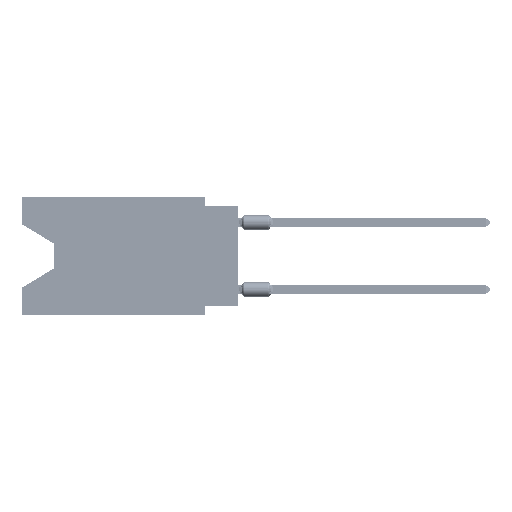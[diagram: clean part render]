
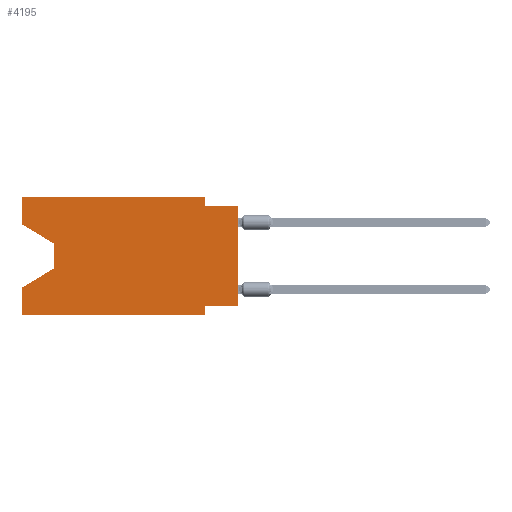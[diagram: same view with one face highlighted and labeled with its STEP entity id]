
A CAD part, left-side view. The second image highlights one B-rep face of the part: STEP entity #4195.
In plain terms, the highlighted planar face has unit normal (-1, 0, 0).
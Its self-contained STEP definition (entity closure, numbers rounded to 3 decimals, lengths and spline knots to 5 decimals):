
#180 = DIRECTION ( 'NONE',  ( 0., -1., 0. ) ) ;
#214 = CARTESIAN_POINT ( 'NONE',  ( 0., 0.645, 0. ) ) ;
#502 = VERTEX_POINT ( 'NONE', #81972 ) ;
#677 = CARTESIAN_POINT ( 'NONE',  ( 0., 0.645, 0. ) ) ;
#2308 = CARTESIAN_POINT ( 'NONE',  ( 0., 0.1, -0.35 ) ) ;
#4195 = ADVANCED_FACE ( 'NONE', ( #60947 ), #52867, .F. ) ;
#5305 = CARTESIAN_POINT ( 'NONE',  ( 0., 0.645, 0. ) ) ;
#5791 = CARTESIAN_POINT ( 'NONE',  ( 0., 0.1, 0. ) ) ;
#6716 = ORIENTED_EDGE ( 'NONE', *, *, #38894, .F. ) ;
#7738 = EDGE_CURVE ( 'NONE', #95306, #88112, #59774, .T. ) ;
#8218 = VECTOR ( 'NONE', #21999, 39.37008 ) ;
#10416 = DIRECTION ( 'NONE',  ( 0., 0., -1. ) ) ;
#10576 = DIRECTION ( 'NONE',  ( 0., -1., 0. ) ) ;
#14417 = LINE ( 'NONE', #21009, #8218 ) ;
#14703 = EDGE_CURVE ( 'NONE', #55074, #41310, #25759, .T. ) ;
#16935 = ORIENTED_EDGE ( 'NONE', *, *, #26205, .T. ) ;
#18198 = LINE ( 'NONE', #49082, #52722 ) ;
#19503 = CARTESIAN_POINT ( 'NONE',  ( 0., 0.55, -0.212 ) ) ;
#21009 = CARTESIAN_POINT ( 'NONE',  ( 0., 0., -0.025 ) ) ;
#21348 = VECTOR ( 'NONE', #34677, 39.37008 ) ;
#21877 = VECTOR ( 'NONE', #88102, 39.37008 ) ;
#21999 = DIRECTION ( 'NONE',  ( 0., -1., 0. ) ) ;
#23014 = CARTESIAN_POINT ( 'NONE',  ( 0., 0.645, -0.35 ) ) ;
#25307 = LINE ( 'NONE', #57171, #21877 ) ;
#25759 = LINE ( 'NONE', #79935, #85732 ) ;
#26205 = EDGE_CURVE ( 'NONE', #72368, #79145, #18198, .T. ) ;
#26707 = VECTOR ( 'NONE', #10416, 39.37008 ) ;
#26899 = CARTESIAN_POINT ( 'NONE',  ( 0., 0.1, 0. ) ) ;
#32857 = DIRECTION ( 'NONE',  ( 0., 0., 1. ) ) ;
#33071 = EDGE_CURVE ( 'NONE', #60863, #79145, #14417, .T. ) ;
#34677 = DIRECTION ( 'NONE',  ( 0., 0., -1. ) ) ;
#36198 = VERTEX_POINT ( 'NONE', #26899 ) ;
#36480 = CARTESIAN_POINT ( 'NONE',  ( 0., 0.645, -0.08025 ) ) ;
#37240 = CARTESIAN_POINT ( 'NONE',  ( 0., 0.645, -0.08025 ) ) ;
#37495 = DIRECTION ( 'NONE',  ( 0., -0.855, -0.519 ) ) ;
#37634 = VERTEX_POINT ( 'NONE', #64694 ) ;
#38363 = EDGE_CURVE ( 'NONE', #72368, #89957, #78567, .T. ) ;
#38894 = EDGE_CURVE ( 'NONE', #95306, #37634, #80423, .T. ) ;
#40051 = CARTESIAN_POINT ( 'NONE',  ( 0., 0., -0.325 ) ) ;
#41310 = VERTEX_POINT ( 'NONE', #59837 ) ;
#42285 = DIRECTION ( 'NONE',  ( 0., 0., 1. ) ) ;
#49082 = CARTESIAN_POINT ( 'NONE',  ( 0., 0., 0. ) ) ;
#49343 = EDGE_CURVE ( 'NONE', #55074, #502, #65061, .T. ) ;
#49981 = CARTESIAN_POINT ( 'NONE',  ( 0., 0.55, -0.138 ) ) ;
#52722 = VECTOR ( 'NONE', #74370, 39.37008 ) ;
#52867 = PLANE ( 'NONE',  #79318 ) ;
#53057 = CARTESIAN_POINT ( 'NONE',  ( 0., 0.1, -0.025 ) ) ;
#53303 = VECTOR ( 'NONE', #42285, 39.37008 ) ;
#53385 = ORIENTED_EDGE ( 'NONE', *, *, #49343, .F. ) ;
#54950 = ORIENTED_EDGE ( 'NONE', *, *, #76757, .T. ) ;
#55024 = ORIENTED_EDGE ( 'NONE', *, *, #33071, .F. ) ;
#55074 = VERTEX_POINT ( 'NONE', #23014 ) ;
#55363 = CARTESIAN_POINT ( 'NONE',  ( 0., 0.55, -0.212 ) ) ;
#55741 = DIRECTION ( 'NONE',  ( 0., 0., -1. ) ) ;
#56237 = ORIENTED_EDGE ( 'NONE', *, *, #38363, .F. ) ;
#56540 = VECTOR ( 'NONE', #180, 39.37008 ) ;
#56626 = CARTESIAN_POINT ( 'NONE',  ( 0., 0.645, 0. ) ) ;
#57171 = CARTESIAN_POINT ( 'NONE',  ( 0., 0.55, -0.138 ) ) ;
#58378 = VERTEX_POINT ( 'NONE', #55363 ) ;
#59080 = CARTESIAN_POINT ( 'NONE',  ( 0., 0., -0.325 ) ) ;
#59774 = LINE ( 'NONE', #36480, #72070 ) ;
#59837 = CARTESIAN_POINT ( 'NONE',  ( 0., 0.1, -0.35 ) ) ;
#60863 = VERTEX_POINT ( 'NONE', #53057 ) ;
#60910 = LINE ( 'NONE', #677, #56540 ) ;
#60947 = FACE_OUTER_BOUND ( 'NONE', #99582, .T. ) ;
#62619 = ORIENTED_EDGE ( 'NONE', *, *, #73472, .F. ) ;
#63772 = ORIENTED_EDGE ( 'NONE', *, *, #14703, .T. ) ;
#64083 = LINE ( 'NONE', #19503, #76512 ) ;
#64555 = VECTOR ( 'NONE', #32857, 39.37008 ) ;
#64694 = CARTESIAN_POINT ( 'NONE',  ( 0., 0.645, 0. ) ) ;
#65061 = LINE ( 'NONE', #5305, #53303 ) ;
#66441 = EDGE_CURVE ( 'NONE', #89957, #41310, #71690, .T. ) ;
#70963 = DIRECTION ( 'NONE',  ( 0., 1., 0. ) ) ;
#71690 = LINE ( 'NONE', #2308, #26707 ) ;
#72070 = VECTOR ( 'NONE', #37495, 39.37008 ) ;
#72368 = VERTEX_POINT ( 'NONE', #59080 ) ;
#72477 = CARTESIAN_POINT ( 'NONE',  ( 0., 0.1, -0.325 ) ) ;
#73472 = EDGE_CURVE ( 'NONE', #37634, #36198, #60910, .T. ) ;
#74370 = DIRECTION ( 'NONE',  ( 0., 0., 1. ) ) ;
#75162 = LINE ( 'NONE', #5791, #21348 ) ;
#76512 = VECTOR ( 'NONE', #88393, 39.37008 ) ;
#76757 = EDGE_CURVE ( 'NONE', #88112, #58378, #25307, .T. ) ;
#78567 = LINE ( 'NONE', #40051, #82288 ) ;
#79145 = VERTEX_POINT ( 'NONE', #89624 ) ;
#79318 = AXIS2_PLACEMENT_3D ( 'NONE', #214, #83761, #55741 ) ;
#79935 = CARTESIAN_POINT ( 'NONE',  ( 0., 0.645, -0.35 ) ) ;
#80423 = LINE ( 'NONE', #56626, #64555 ) ;
#81972 = CARTESIAN_POINT ( 'NONE',  ( 0., 0.645, -0.26975 ) ) ;
#82288 = VECTOR ( 'NONE', #70963, 39.37008 ) ;
#83761 = DIRECTION ( 'NONE',  ( 1., 0., 0. ) ) ;
#85732 = VECTOR ( 'NONE', #10576, 39.37008 ) ;
#86659 = ORIENTED_EDGE ( 'NONE', *, *, #98401, .F. ) ;
#88102 = DIRECTION ( 'NONE',  ( 0., 0., -1. ) ) ;
#88112 = VERTEX_POINT ( 'NONE', #49981 ) ;
#88393 = DIRECTION ( 'NONE',  ( 0., 0.855, -0.519 ) ) ;
#89111 = ORIENTED_EDGE ( 'NONE', *, *, #99472, .T. ) ;
#89408 = ORIENTED_EDGE ( 'NONE', *, *, #66441, .F. ) ;
#89624 = CARTESIAN_POINT ( 'NONE',  ( 0., 0., -0.025 ) ) ;
#89957 = VERTEX_POINT ( 'NONE', #72477 ) ;
#95306 = VERTEX_POINT ( 'NONE', #37240 ) ;
#95512 = ORIENTED_EDGE ( 'NONE', *, *, #7738, .T. ) ;
#98401 = EDGE_CURVE ( 'NONE', #36198, #60863, #75162, .T. ) ;
#99472 = EDGE_CURVE ( 'NONE', #58378, #502, #64083, .T. ) ;
#99582 = EDGE_LOOP ( 'NONE', ( #95512, #54950, #89111, #53385, #63772, #89408, #56237, #16935, #55024, #86659, #62619, #6716 ) ) ;
